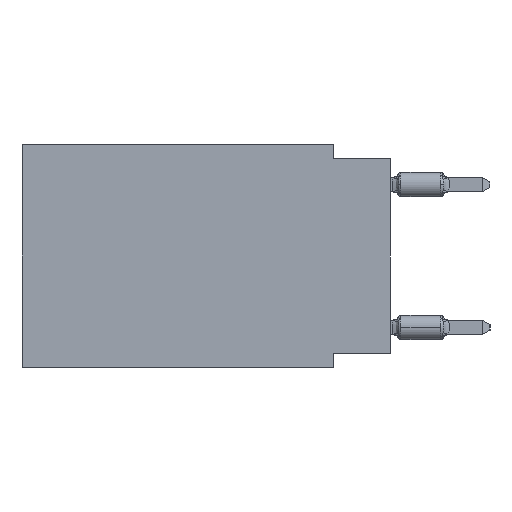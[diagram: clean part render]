
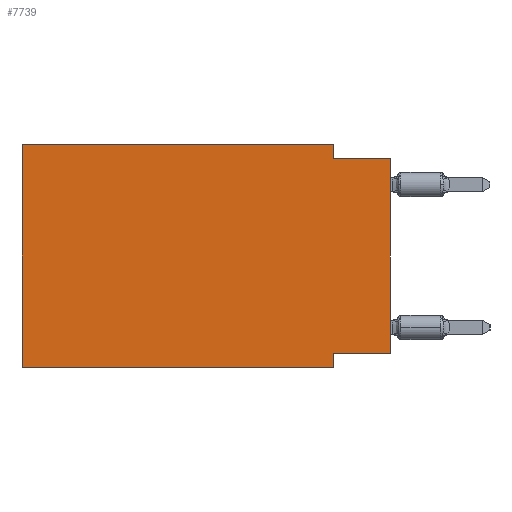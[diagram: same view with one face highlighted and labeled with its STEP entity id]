
A CAD part, left-side view. The second image highlights one B-rep face of the part: STEP entity #7739.
In plain terms, the highlighted planar face has unit normal (-1, 0, 0).
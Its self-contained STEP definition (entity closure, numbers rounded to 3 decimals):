
#236 = VERTEX_POINT ( 'NONE', #32292 ) ;
#252 = DIRECTION ( 'NONE',  ( 0., -1., 0. ) ) ;
#668 = LINE ( 'NONE', #38611, #17196 ) ;
#703 = CARTESIAN_POINT ( 'NONE',  ( 0., 2.54, -0.635 ) ) ;
#844 = DIRECTION ( 'NONE',  ( 0., 0., -1. ) ) ;
#864 = VERTEX_POINT ( 'NONE', #17308 ) ;
#2323 = VECTOR ( 'NONE', #2986, 1000. ) ;
#2425 = CARTESIAN_POINT ( 'NONE',  ( 0., 16.383, 0. ) ) ;
#2492 = VECTOR ( 'NONE', #28535, 1000. ) ;
#2986 = DIRECTION ( 'NONE',  ( 0., -1., 0. ) ) ;
#4303 = LINE ( 'NONE', #16939, #17312 ) ;
#4707 = DIRECTION ( 'NONE',  ( 0., 0., -1. ) ) ;
#4727 = VERTEX_POINT ( 'NONE', #39393 ) ;
#5536 = PLANE ( 'NONE',  #14080 ) ;
#6496 = VECTOR ( 'NONE', #27292, 1000. ) ;
#7503 = CARTESIAN_POINT ( 'NONE',  ( 0., 16.383, -9.906 ) ) ;
#7739 = ADVANCED_FACE ( 'NONE', ( #33935 ), #5536, .F. ) ;
#8417 = CARTESIAN_POINT ( 'NONE',  ( 0., 2.54, -9.271 ) ) ;
#10534 = VERTEX_POINT ( 'NONE', #7503 ) ;
#10944 = ORIENTED_EDGE ( 'NONE', *, *, #40928, .F. ) ;
#11378 = ORIENTED_EDGE ( 'NONE', *, *, #36453, .T. ) ;
#11525 = LINE ( 'NONE', #36022, #6496 ) ;
#12350 = DIRECTION ( 'NONE',  ( 0., 0., 1. ) ) ;
#13478 = LINE ( 'NONE', #32562, #20287 ) ;
#14080 = AXIS2_PLACEMENT_3D ( 'NONE', #2425, #31245, #21895 ) ;
#15474 = EDGE_CURVE ( 'NONE', #29638, #236, #13478, .T. ) ;
#15751 = ORIENTED_EDGE ( 'NONE', *, *, #19034, .F. ) ;
#16939 = CARTESIAN_POINT ( 'NONE',  ( 0., 2.54, 0. ) ) ;
#17196 = VECTOR ( 'NONE', #252, 1000. ) ;
#17308 = CARTESIAN_POINT ( 'NONE',  ( 0., 0., -9.271 ) ) ;
#17312 = VECTOR ( 'NONE', #4707, 1000. ) ;
#17742 = ORIENTED_EDGE ( 'NONE', *, *, #29693, .T. ) ;
#18163 = VECTOR ( 'NONE', #12350, 1000. ) ;
#18737 = LINE ( 'NONE', #31397, #2323 ) ;
#19034 = EDGE_CURVE ( 'NONE', #34769, #29449, #668, .T. ) ;
#19240 = CARTESIAN_POINT ( 'NONE',  ( 0., 2.54, 0. ) ) ;
#20276 = VECTOR ( 'NONE', #36005, 1000. ) ;
#20287 = VECTOR ( 'NONE', #844, 1000. ) ;
#20634 = LINE ( 'NONE', #23344, #20276 ) ;
#21166 = EDGE_CURVE ( 'NONE', #29449, #32275, #4303, .T. ) ;
#21895 = DIRECTION ( 'NONE',  ( 0., 0., -1. ) ) ;
#22090 = CARTESIAN_POINT ( 'NONE',  ( 0., 0., -0.635 ) ) ;
#22259 = ORIENTED_EDGE ( 'NONE', *, *, #21166, .F. ) ;
#23344 = CARTESIAN_POINT ( 'NONE',  ( 0., 16.383, 0. ) ) ;
#24500 = CARTESIAN_POINT ( 'NONE',  ( 0., 16.383, 0. ) ) ;
#25211 = LINE ( 'NONE', #22090, #2492 ) ;
#27121 = ORIENTED_EDGE ( 'NONE', *, *, #15474, .F. ) ;
#27292 = DIRECTION ( 'NONE',  ( 0., 1., 0. ) ) ;
#28527 = LINE ( 'NONE', #37662, #18163 ) ;
#28535 = DIRECTION ( 'NONE',  ( 0., -1., 0. ) ) ;
#29449 = VERTEX_POINT ( 'NONE', #19240 ) ;
#29638 = VERTEX_POINT ( 'NONE', #8417 ) ;
#29693 = EDGE_CURVE ( 'NONE', #864, #4727, #28527, .T. ) ;
#31245 = DIRECTION ( 'NONE',  ( 1., 0., 0. ) ) ;
#31397 = CARTESIAN_POINT ( 'NONE',  ( 0., 16.383, -9.906 ) ) ;
#31780 = EDGE_CURVE ( 'NONE', #32275, #4727, #25211, .T. ) ;
#32275 = VERTEX_POINT ( 'NONE', #703 ) ;
#32292 = CARTESIAN_POINT ( 'NONE',  ( 0., 2.54, -9.906 ) ) ;
#32562 = CARTESIAN_POINT ( 'NONE',  ( 0., 2.54, -9.906 ) ) ;
#32579 = EDGE_LOOP ( 'NONE', ( #17742, #35108, #22259, #15751, #38776, #11378, #27121, #10944 ) ) ;
#33935 = FACE_OUTER_BOUND ( 'NONE', #32579, .T. ) ;
#34769 = VERTEX_POINT ( 'NONE', #24500 ) ;
#35108 = ORIENTED_EDGE ( 'NONE', *, *, #31780, .F. ) ;
#36005 = DIRECTION ( 'NONE',  ( 0., 0., 1. ) ) ;
#36022 = CARTESIAN_POINT ( 'NONE',  ( 0., 0., -9.271 ) ) ;
#36453 = EDGE_CURVE ( 'NONE', #10534, #236, #18737, .T. ) ;
#37421 = EDGE_CURVE ( 'NONE', #10534, #34769, #20634, .T. ) ;
#37662 = CARTESIAN_POINT ( 'NONE',  ( 0., 0., 0. ) ) ;
#38611 = CARTESIAN_POINT ( 'NONE',  ( 0., 16.383, 0. ) ) ;
#38776 = ORIENTED_EDGE ( 'NONE', *, *, #37421, .F. ) ;
#39393 = CARTESIAN_POINT ( 'NONE',  ( 0., 0., -0.635 ) ) ;
#40928 = EDGE_CURVE ( 'NONE', #864, #29638, #11525, .T. ) ;
